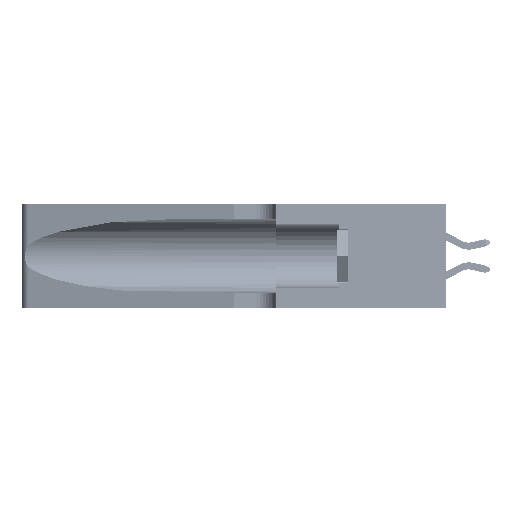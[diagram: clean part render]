
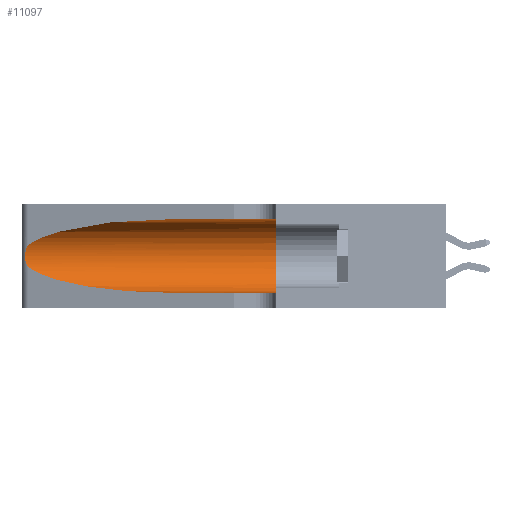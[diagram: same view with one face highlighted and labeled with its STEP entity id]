
A CAD part, left-side view. The second image highlights one B-rep face of the part: STEP entity #11097.
In plain terms, the highlighted cylindrical face has radius 3.308 mm (diameter 6.617 mm), a partial arc.
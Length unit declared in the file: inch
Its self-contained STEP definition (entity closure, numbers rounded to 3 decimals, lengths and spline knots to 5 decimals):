
#403 = CARTESIAN_POINT ( 'NONE',  ( 0.25487, 1.22718, 0.22369 ) ) ;
#2962 = ORIENTED_EDGE ( 'NONE', *, *, #34666, .F. ) ;
#3700 = CARTESIAN_POINT ( 'NONE',  ( 0.18966, 0.96281, 0.05475 ) ) ;
#6287 = EDGE_CURVE ( 'NONE', #6391, #21725, #17370, .T. ) ;
#6391 = VERTEX_POINT ( 'NONE', #36855 ) ;
#6437 = DIRECTION ( 'NONE',  ( 0., 1., 0. ) ) ;
#6526 = FACE_OUTER_BOUND ( 'NONE', #12724, .T. ) ;
#7253 = CARTESIAN_POINT ( 'NONE',  ( 0.25787, 1.23484, 0.2124 ) ) ;
#10460 = VERTEX_POINT ( 'NONE', #21972 ) ;
#11097 = ADVANCED_FACE ( 'NONE', ( #6526 ), #27217, .F. ) ;
#11434 = CARTESIAN_POINT ( 'NONE',  ( 0.26018, 1.23835, 0.19895 ) ) ;
#12724 = EDGE_LOOP ( 'NONE', ( #16049, #46940, #32878, #36705, #51386, #2962 ) ) ;
#13424 = DIRECTION ( 'NONE',  ( 0., 0., -1. ) ) ;
#14160 = VECTOR ( 'NONE', #50045, 39.37008 ) ;
#15565 = CARTESIAN_POINT ( 'NONE',  ( 0.26075, 1.23896, 0.178 ) ) ;
#15762 = LINE ( 'NONE', #16075, #47382 ) ;
#16049 = ORIENTED_EDGE ( 'NONE', *, *, #37471, .T. ) ;
#16075 = CARTESIAN_POINT ( 'NONE',  ( 0.1305, 1.61858, 0.31525 ) ) ;
#17370 = B_SPLINE_CURVE_WITH_KNOTS ( 'NONE', 3,
 ( #31993, #52543, #35957, #7253, #36141, #11434, #40296, #15565, #44421, #19714, #48575, #23882, #52723, #28031 ),
 .UNSPECIFIED., .F., .F.,
 ( 4, 2, 2, 2, 2, 2, 4 ),
 ( 0., 0.00027, 0.00053, 0.00107, 0.0016, 0.00187, 0.00214 ),
 .UNSPECIFIED. ) ;
#17388 = DIRECTION ( 'NONE',  ( 0., -1., 0. ) ) ;
#19714 = CARTESIAN_POINT ( 'NONE',  ( 0.25856, 1.23593, 0.16098 ) ) ;
#20166 = CARTESIAN_POINT ( 'NONE',  ( 0.2373, 1.15595, 0.08982 ) ) ;
#20213 = DIRECTION ( 'NONE',  ( 0., -1., 0. ) ) ;
#21085 = CARTESIAN_POINT ( 'NONE',  ( 0.1305, 0.72297, 0.31525 ) ) ;
#21351 =( BOUNDED_CURVE ( )  B_SPLINE_CURVE ( 3, ( #53159, #20166, #3700, #32631 ),
 .UNSPECIFIED., .F., .F. ) 
 B_SPLINE_CURVE_WITH_KNOTS ( ( 4, 4 ),
 ( 3.44316, 4.71239 ),
 .UNSPECIFIED. ) 
 CURVE ( )  GEOMETRIC_REPRESENTATION_ITEM ( )  RATIONAL_B_SPLINE_CURVE ( ( 1., 0.87, 0.87, 1. ) ) 
 REPRESENTATION_ITEM ( '' )  );
#21725 = VERTEX_POINT ( 'NONE', #31282 ) ;
#21972 = CARTESIAN_POINT ( 'NONE',  ( 0.1305, 0.72297, 0.31525 ) ) ;
#23695 = CARTESIAN_POINT ( 'NONE',  ( 0.1305, 0.35, 0.05475 ) ) ;
#23882 = CARTESIAN_POINT ( 'NONE',  ( 0.25639, 1.23186, 0.15144 ) ) ;
#25141 = LINE ( 'NONE', #49865, #14160 ) ;
#25255 = CARTESIAN_POINT ( 'NONE',  ( 0.2373, 1.15595, 0.28018 ) ) ;
#27016 =( BOUNDED_CURVE ( )  B_SPLINE_CURVE ( 3, ( #21085, #37518, #25255, #403 ),
 .UNSPECIFIED., .F., .F. ) 
 B_SPLINE_CURVE_WITH_KNOTS ( ( 4, 4 ),
 ( 1.5708, 2.84003 ),
 .UNSPECIFIED. ) 
 CURVE ( )  GEOMETRIC_REPRESENTATION_ITEM ( )  RATIONAL_B_SPLINE_CURVE ( ( 1., 0.87, 0.87, 1. ) ) 
 REPRESENTATION_ITEM ( '' )  );
#27217 = CYLINDRICAL_SURFACE ( 'NONE', #41076, 0.13025 ) ;
#28031 = CARTESIAN_POINT ( 'NONE',  ( 0.25487, 1.22718, 0.14631 ) ) ;
#29107 = EDGE_CURVE ( 'NONE', #21725, #39890, #21351, .T. ) ;
#31172 = CARTESIAN_POINT ( 'NONE',  ( 0.1305, 0.35, 0.185 ) ) ;
#31282 = CARTESIAN_POINT ( 'NONE',  ( 0.25487, 1.22718, 0.14631 ) ) ;
#31993 = CARTESIAN_POINT ( 'NONE',  ( 0.25487, 1.22718, 0.22369 ) ) ;
#32631 = CARTESIAN_POINT ( 'NONE',  ( 0.1305, 0.72297, 0.05475 ) ) ;
#32878 = ORIENTED_EDGE ( 'NONE', *, *, #29107, .T. ) ;
#34666 = EDGE_CURVE ( 'NONE', #10460, #38048, #15762, .T. ) ;
#34969 = AXIS2_PLACEMENT_3D ( 'NONE', #31172, #6437, #35308 ) ;
#35308 = DIRECTION ( 'NONE',  ( 0., 0., 1. ) ) ;
#35957 = CARTESIAN_POINT ( 'NONE',  ( 0.25639, 1.23184, 0.21858 ) ) ;
#36141 = CARTESIAN_POINT ( 'NONE',  ( 0.25854, 1.2359, 0.20912 ) ) ;
#36705 = ORIENTED_EDGE ( 'NONE', *, *, #47454, .T. ) ;
#36855 = CARTESIAN_POINT ( 'NONE',  ( 0.25487, 1.22718, 0.22369 ) ) ;
#37471 = EDGE_CURVE ( 'NONE', #10460, #6391, #27016, .T. ) ;
#37518 = CARTESIAN_POINT ( 'NONE',  ( 0.18966, 0.96281, 0.31525 ) ) ;
#38048 = VERTEX_POINT ( 'NONE', #49715 ) ;
#38152 = CARTESIAN_POINT ( 'NONE',  ( 0.1305, 1.61858, 0.185 ) ) ;
#39890 = VERTEX_POINT ( 'NONE', #49198 ) ;
#40296 = CARTESIAN_POINT ( 'NONE',  ( 0.26075, 1.23896, 0.19203 ) ) ;
#41076 = AXIS2_PLACEMENT_3D ( 'NONE', #38152, #17388, #13424 ) ;
#44421 = CARTESIAN_POINT ( 'NONE',  ( 0.26017, 1.23833, 0.17102 ) ) ;
#46940 = ORIENTED_EDGE ( 'NONE', *, *, #6287, .T. ) ;
#47382 = VECTOR ( 'NONE', #20213, 39.37008 ) ;
#47454 = EDGE_CURVE ( 'NONE', #39890, #47891, #25141, .T. ) ;
#47540 = CIRCLE ( 'NONE', #34969, 0.13025 ) ;
#47891 = VERTEX_POINT ( 'NONE', #23695 ) ;
#48575 = CARTESIAN_POINT ( 'NONE',  ( 0.25789, 1.23486, 0.15765 ) ) ;
#49046 = EDGE_CURVE ( 'NONE', #38048, #47891, #47540, .T. ) ;
#49198 = CARTESIAN_POINT ( 'NONE',  ( 0.1305, 0.72297, 0.05475 ) ) ;
#49715 = CARTESIAN_POINT ( 'NONE',  ( 0.1305, 0.35, 0.31525 ) ) ;
#49865 = CARTESIAN_POINT ( 'NONE',  ( 0.1305, 1.61858, 0.05475 ) ) ;
#50045 = DIRECTION ( 'NONE',  ( 0., -1., 0. ) ) ;
#51386 = ORIENTED_EDGE ( 'NONE', *, *, #49046, .F. ) ;
#52543 = CARTESIAN_POINT ( 'NONE',  ( 0.25555, 1.22994, 0.2215 ) ) ;
#52723 = CARTESIAN_POINT ( 'NONE',  ( 0.25555, 1.22993, 0.14849 ) ) ;
#53159 = CARTESIAN_POINT ( 'NONE',  ( 0.25487, 1.22718, 0.14631 ) ) ;
